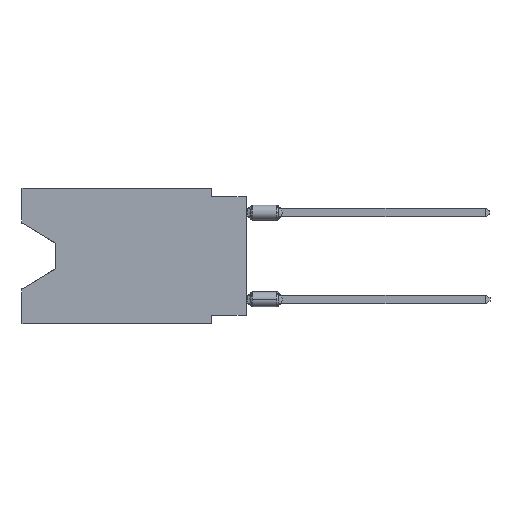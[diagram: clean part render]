
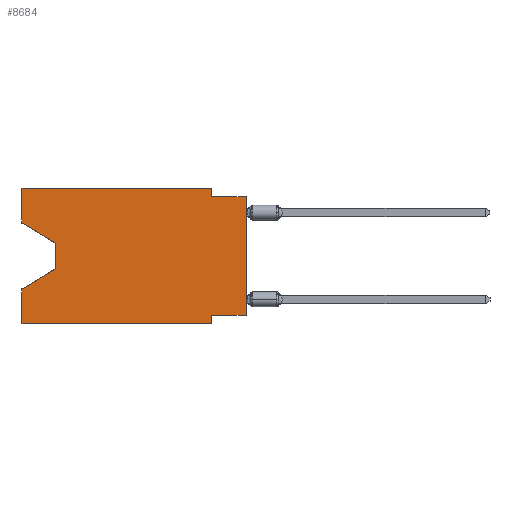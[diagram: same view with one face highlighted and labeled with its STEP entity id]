
A CAD part, left-side view. The second image highlights one B-rep face of the part: STEP entity #8684.
In plain terms, the highlighted planar face has unit normal (-1, 0, 0).
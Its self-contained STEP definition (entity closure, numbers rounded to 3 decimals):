
#43 = DIRECTION ( 'NONE',  ( 0., -1., 0. ) ) ;
#64 = DIRECTION ( 'NONE',  ( 0., -1., 0. ) ) ;
#824 = DIRECTION ( 'NONE',  ( 0., -0.855, -0.519 ) ) ;
#1057 = ORIENTED_EDGE ( 'NONE', *, *, #19632, .F. ) ;
#1212 = FACE_OUTER_BOUND ( 'NONE', #5663, .T. ) ;
#1232 = DIRECTION ( 'NONE',  ( 0., 0., -1. ) ) ;
#1584 = VECTOR ( 'NONE', #4762, 1000. ) ;
#1984 = DIRECTION ( 'NONE',  ( 0., 1., 0. ) ) ;
#2099 = DIRECTION ( 'NONE',  ( 0., 0.855, -0.519 ) ) ;
#2619 = DIRECTION ( 'NONE',  ( 0., 0., -1. ) ) ;
#2701 = EDGE_CURVE ( 'NONE', #3683, #10244, #3319, .T. ) ;
#2771 = EDGE_CURVE ( 'NONE', #10800, #18586, #12808, .T. ) ;
#2863 = LINE ( 'NONE', #7628, #14374 ) ;
#3105 = CARTESIAN_POINT ( 'NONE',  ( 0., 16.383, -7.36 ) ) ;
#3319 = LINE ( 'NONE', #15643, #16481 ) ;
#3332 = ORIENTED_EDGE ( 'NONE', *, *, #2771, .T. ) ;
#3608 = CARTESIAN_POINT ( 'NONE',  ( 0., 0., -9.271 ) ) ;
#3617 = CARTESIAN_POINT ( 'NONE',  ( 0., 13.97, -5.893 ) ) ;
#3683 = VERTEX_POINT ( 'NONE', #9850 ) ;
#3826 = CARTESIAN_POINT ( 'NONE',  ( 0., 2.54, 0. ) ) ;
#4102 = ORIENTED_EDGE ( 'NONE', *, *, #2701, .T. ) ;
#4261 = EDGE_CURVE ( 'NONE', #8078, #15122, #9923, .T. ) ;
#4539 = EDGE_CURVE ( 'NONE', #15122, #10800, #9299, .T. ) ;
#4551 = VECTOR ( 'NONE', #824, 1000. ) ;
#4762 = DIRECTION ( 'NONE',  ( 0., 0., -1. ) ) ;
#4788 = EDGE_CURVE ( 'NONE', #7972, #10173, #16950, .T. ) ;
#5509 = ORIENTED_EDGE ( 'NONE', *, *, #4788, .F. ) ;
#5591 = CARTESIAN_POINT ( 'NONE',  ( 0., 16.383, -9.906 ) ) ;
#5663 = EDGE_LOOP ( 'NONE', ( #15772, #17739, #3332, #13219, #6973, #13740, #1057, #4102, #19943, #19510, #5509, #7552 ) ) ;
#5902 = LINE ( 'NONE', #18459, #16291 ) ;
#6097 = AXIS2_PLACEMENT_3D ( 'NONE', #10296, #16471, #2619 ) ;
#6301 = EDGE_CURVE ( 'NONE', #19919, #10244, #2863, .T. ) ;
#6320 = CARTESIAN_POINT ( 'NONE',  ( 0., 16.383, 0. ) ) ;
#6516 = EDGE_CURVE ( 'NONE', #9813, #11012, #19628, .T. ) ;
#6860 = CARTESIAN_POINT ( 'NONE',  ( 0., 2.54, -9.906 ) ) ;
#6973 = ORIENTED_EDGE ( 'NONE', *, *, #13613, .T. ) ;
#7154 = EDGE_CURVE ( 'NONE', #10173, #19919, #14055, .T. ) ;
#7357 = CARTESIAN_POINT ( 'NONE',  ( 0., 16.383, -9.906 ) ) ;
#7481 = VECTOR ( 'NONE', #10185, 1000. ) ;
#7552 = ORIENTED_EDGE ( 'NONE', *, *, #12024, .F. ) ;
#7628 = CARTESIAN_POINT ( 'NONE',  ( 0., 0., -0.635 ) ) ;
#7729 = CARTESIAN_POINT ( 'NONE',  ( 0., 16.383, 0. ) ) ;
#7972 = VERTEX_POINT ( 'NONE', #7729 ) ;
#8078 = VERTEX_POINT ( 'NONE', #8509 ) ;
#8509 = CARTESIAN_POINT ( 'NONE',  ( 0., 16.383, -2.546 ) ) ;
#8684 = ADVANCED_FACE ( 'NONE', ( #1212 ), #18089, .F. ) ;
#9000 = CARTESIAN_POINT ( 'NONE',  ( 0., 2.54, 0. ) ) ;
#9299 = LINE ( 'NONE', #19080, #10339 ) ;
#9813 = VERTEX_POINT ( 'NONE', #11525 ) ;
#9850 = CARTESIAN_POINT ( 'NONE',  ( 0., 0., -9.271 ) ) ;
#9923 = LINE ( 'NONE', #16489, #4551 ) ;
#9959 = LINE ( 'NONE', #3608, #14330 ) ;
#10173 = VERTEX_POINT ( 'NONE', #3826 ) ;
#10185 = DIRECTION ( 'NONE',  ( 0., -1., 0. ) ) ;
#10244 = VERTEX_POINT ( 'NONE', #13207 ) ;
#10296 = CARTESIAN_POINT ( 'NONE',  ( 0., 16.383, 0. ) ) ;
#10339 = VECTOR ( 'NONE', #15833, 1000. ) ;
#10453 = CARTESIAN_POINT ( 'NONE',  ( 0., 13.97, -5.893 ) ) ;
#10800 = VERTEX_POINT ( 'NONE', #10453 ) ;
#11012 = VERTEX_POINT ( 'NONE', #6860 ) ;
#11525 = CARTESIAN_POINT ( 'NONE',  ( 0., 2.54, -9.271 ) ) ;
#12024 = EDGE_CURVE ( 'NONE', #8078, #7972, #18199, .T. ) ;
#12775 = DIRECTION ( 'NONE',  ( 0., 0., 1. ) ) ;
#12808 = LINE ( 'NONE', #3617, #17454 ) ;
#13207 = CARTESIAN_POINT ( 'NONE',  ( 0., 0., -0.635 ) ) ;
#13219 = ORIENTED_EDGE ( 'NONE', *, *, #17940, .F. ) ;
#13416 = LINE ( 'NONE', #7357, #7481 ) ;
#13613 = EDGE_CURVE ( 'NONE', #17026, #11012, #13416, .T. ) ;
#13740 = ORIENTED_EDGE ( 'NONE', *, *, #6516, .F. ) ;
#14055 = LINE ( 'NONE', #9000, #1584 ) ;
#14330 = VECTOR ( 'NONE', #1984, 1000. ) ;
#14374 = VECTOR ( 'NONE', #43, 1000. ) ;
#15122 = VERTEX_POINT ( 'NONE', #17519 ) ;
#15260 = DIRECTION ( 'NONE',  ( 0., 0., 1. ) ) ;
#15643 = CARTESIAN_POINT ( 'NONE',  ( 0., 0., 0. ) ) ;
#15772 = ORIENTED_EDGE ( 'NONE', *, *, #4261, .T. ) ;
#15833 = DIRECTION ( 'NONE',  ( 0., 0., -1. ) ) ;
#16291 = VECTOR ( 'NONE', #12775, 1000. ) ;
#16471 = DIRECTION ( 'NONE',  ( 1., 0., 0. ) ) ;
#16481 = VECTOR ( 'NONE', #17364, 1000. ) ;
#16489 = CARTESIAN_POINT ( 'NONE',  ( 0., 16.383, -2.546 ) ) ;
#16950 = LINE ( 'NONE', #6320, #17867 ) ;
#17026 = VERTEX_POINT ( 'NONE', #5591 ) ;
#17364 = DIRECTION ( 'NONE',  ( 0., 0., 1. ) ) ;
#17454 = VECTOR ( 'NONE', #2099, 1000. ) ;
#17519 = CARTESIAN_POINT ( 'NONE',  ( 0., 13.97, -4.013 ) ) ;
#17739 = ORIENTED_EDGE ( 'NONE', *, *, #4539, .T. ) ;
#17867 = VECTOR ( 'NONE', #64, 1000. ) ;
#17940 = EDGE_CURVE ( 'NONE', #17026, #18586, #5902, .T. ) ;
#18089 = PLANE ( 'NONE',  #6097 ) ;
#18101 = VECTOR ( 'NONE', #15260, 1000. ) ;
#18199 = LINE ( 'NONE', #19708, #18101 ) ;
#18269 = VECTOR ( 'NONE', #1232, 1000. ) ;
#18459 = CARTESIAN_POINT ( 'NONE',  ( 0., 16.383, 0. ) ) ;
#18586 = VERTEX_POINT ( 'NONE', #3105 ) ;
#19080 = CARTESIAN_POINT ( 'NONE',  ( 0., 13.97, -4.013 ) ) ;
#19510 = ORIENTED_EDGE ( 'NONE', *, *, #7154, .F. ) ;
#19531 = CARTESIAN_POINT ( 'NONE',  ( 0., 2.54, -9.906 ) ) ;
#19628 = LINE ( 'NONE', #19531, #18269 ) ;
#19632 = EDGE_CURVE ( 'NONE', #3683, #9813, #9959, .T. ) ;
#19708 = CARTESIAN_POINT ( 'NONE',  ( 0., 16.383, 0. ) ) ;
#19767 = CARTESIAN_POINT ( 'NONE',  ( 0., 2.54, -0.635 ) ) ;
#19919 = VERTEX_POINT ( 'NONE', #19767 ) ;
#19943 = ORIENTED_EDGE ( 'NONE', *, *, #6301, .F. ) ;
